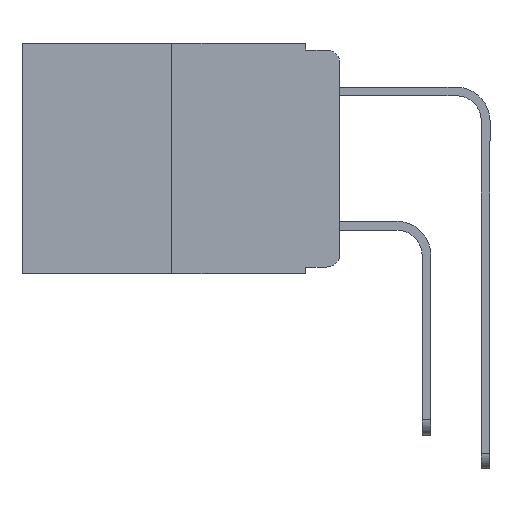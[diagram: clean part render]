
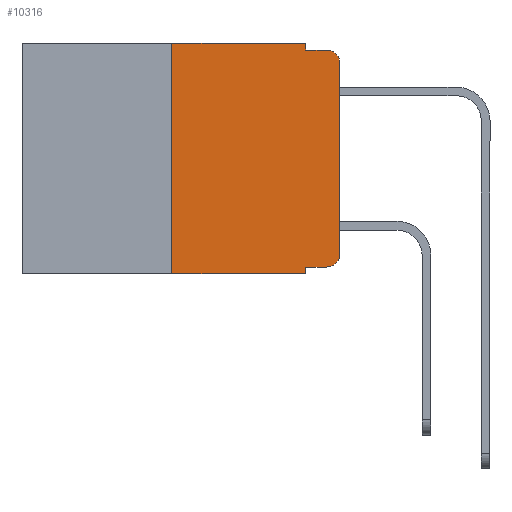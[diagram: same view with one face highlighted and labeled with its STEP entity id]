
A CAD part, left-side view. The second image highlights one B-rep face of the part: STEP entity #10316.
In plain terms, the highlighted planar face has unit normal (-1, 0, 0).
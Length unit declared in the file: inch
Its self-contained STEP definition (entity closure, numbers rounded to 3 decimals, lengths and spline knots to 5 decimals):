
#369 = LINE ( 'NONE', #493, #10922 ) ;
#422 = VERTEX_POINT ( 'NONE', #744 ) ;
#456 = CARTESIAN_POINT ( 'NONE',  ( 0., 0.051, -0.01 ) ) ;
#493 = CARTESIAN_POINT ( 'NONE',  ( 0., 0.473, 0. ) ) ;
#635 = EDGE_CURVE ( 'NONE', #11905, #3567, #12122, .T. ) ;
#669 = LINE ( 'NONE', #4053, #11160 ) ;
#709 = VERTEX_POINT ( 'NONE', #1721 ) ;
#716 = VERTEX_POINT ( 'NONE', #5108 ) ;
#744 = CARTESIAN_POINT ( 'NONE',  ( 0., 0.051, -0.343 ) ) ;
#819 = DIRECTION ( 'NONE',  ( 0., -1., 0. ) ) ;
#1115 = CARTESIAN_POINT ( 'NONE',  ( 0., 0.473, 0. ) ) ;
#1417 = DIRECTION ( 'NONE',  ( 0., 0., 1. ) ) ;
#1721 = CARTESIAN_POINT ( 'NONE',  ( 0., 0., -0.313 ) ) ;
#1828 = DIRECTION ( 'NONE',  ( 0., 0., -1. ) ) ;
#1864 = DIRECTION ( 'NONE',  ( -1., 0., 0. ) ) ;
#1918 = CARTESIAN_POINT ( 'NONE',  ( 0., 0.473, -0.343 ) ) ;
#2190 = DIRECTION ( 'NONE',  ( 0., -1., 0. ) ) ;
#2200 = PLANE ( 'NONE',  #5521 ) ;
#2297 = CIRCLE ( 'NONE', #5260, 0.02 ) ;
#2312 = VECTOR ( 'NONE', #10658, 39.37008 ) ;
#2382 = DIRECTION ( 'NONE',  ( 0., 0., -1. ) ) ;
#2563 = FACE_OUTER_BOUND ( 'NONE', #3413, .T. ) ;
#2574 = ORIENTED_EDGE ( 'NONE', *, *, #4905, .F. ) ;
#2750 = ORIENTED_EDGE ( 'NONE', *, *, #12150, .F. ) ;
#2916 = CARTESIAN_POINT ( 'NONE',  ( 0., 0.051, 0. ) ) ;
#3266 = ORIENTED_EDGE ( 'NONE', *, *, #9409, .F. ) ;
#3413 = EDGE_LOOP ( 'NONE', ( #11292, #5537, #2574, #2750, #3266, #3460, #7103, #6389, #4640, #3563 ) ) ;
#3460 = ORIENTED_EDGE ( 'NONE', *, *, #635, .F. ) ;
#3563 = ORIENTED_EDGE ( 'NONE', *, *, #5731, .T. ) ;
#3567 = VERTEX_POINT ( 'NONE', #7521 ) ;
#4053 = CARTESIAN_POINT ( 'NONE',  ( 0., 0.051, 0. ) ) ;
#4135 = LINE ( 'NONE', #1918, #9177 ) ;
#4256 = DIRECTION ( 'NONE',  ( 1., 0., 0. ) ) ;
#4304 = DIRECTION ( 'NONE',  ( 0., 0., 1. ) ) ;
#4493 = CARTESIAN_POINT ( 'NONE',  ( 0., 0.02, -0.03 ) ) ;
#4640 = ORIENTED_EDGE ( 'NONE', *, *, #7747, .T. ) ;
#4781 = DIRECTION ( 'NONE',  ( 0., -1., 0. ) ) ;
#4905 = EDGE_CURVE ( 'NONE', #8538, #7505, #7446, .T. ) ;
#5053 = CARTESIAN_POINT ( 'NONE',  ( 0., 0.02, -0.333 ) ) ;
#5089 = VECTOR ( 'NONE', #2382, 39.37008 ) ;
#5108 = CARTESIAN_POINT ( 'NONE',  ( 0., 0., -0.03 ) ) ;
#5260 = AXIS2_PLACEMENT_3D ( 'NONE', #4493, #11409, #5527 ) ;
#5336 = CARTESIAN_POINT ( 'NONE',  ( 0., 0., 0. ) ) ;
#5478 = EDGE_CURVE ( 'NONE', #12094, #422, #12902, .T. ) ;
#5521 = AXIS2_PLACEMENT_3D ( 'NONE', #1115, #4256, #9312 ) ;
#5527 = DIRECTION ( 'NONE',  ( 0., 0., -1. ) ) ;
#5537 = ORIENTED_EDGE ( 'NONE', *, *, #8377, .T. ) ;
#5731 = EDGE_CURVE ( 'NONE', #9114, #709, #10222, .T. ) ;
#6389 = ORIENTED_EDGE ( 'NONE', *, *, #5478, .F. ) ;
#6400 = CARTESIAN_POINT ( 'NONE',  ( 0., 0.02, -0.313 ) ) ;
#7103 = ORIENTED_EDGE ( 'NONE', *, *, #7580, .T. ) ;
#7446 = LINE ( 'NONE', #456, #2312 ) ;
#7505 = VERTEX_POINT ( 'NONE', #11778 ) ;
#7521 = CARTESIAN_POINT ( 'NONE',  ( 0., 0.25, 0. ) ) ;
#7556 = VERTEX_POINT ( 'NONE', #9016 ) ;
#7580 = EDGE_CURVE ( 'NONE', #11905, #422, #4135, .T. ) ;
#7747 = EDGE_CURVE ( 'NONE', #12094, #9114, #10820, .T. ) ;
#8141 = CARTESIAN_POINT ( 'NONE',  ( 0., 0.25, 0. ) ) ;
#8377 = EDGE_CURVE ( 'NONE', #716, #7505, #2297, .T. ) ;
#8538 = VERTEX_POINT ( 'NONE', #9751 ) ;
#9016 = CARTESIAN_POINT ( 'NONE',  ( 0., 0.051, 0. ) ) ;
#9114 = VERTEX_POINT ( 'NONE', #5053 ) ;
#9177 = VECTOR ( 'NONE', #819, 39.37008 ) ;
#9312 = DIRECTION ( 'NONE',  ( 0., 0., -1. ) ) ;
#9409 = EDGE_CURVE ( 'NONE', #3567, #7556, #369, .T. ) ;
#9589 = CARTESIAN_POINT ( 'NONE',  ( 0., 0.25, -0.343 ) ) ;
#9590 = VECTOR ( 'NONE', #1417, 39.37008 ) ;
#9751 = CARTESIAN_POINT ( 'NONE',  ( 0., 0.051, -0.01 ) ) ;
#9929 = VECTOR ( 'NONE', #2190, 39.37008 ) ;
#10222 = CIRCLE ( 'NONE', #11117, 0.02 ) ;
#10305 = VECTOR ( 'NONE', #4304, 39.37008 ) ;
#10316 = ADVANCED_FACE ( 'NONE', ( #2563 ), #2200, .F. ) ;
#10331 = EDGE_CURVE ( 'NONE', #709, #716, #12822, .T. ) ;
#10658 = DIRECTION ( 'NONE',  ( 0., -1., 0. ) ) ;
#10820 = LINE ( 'NONE', #13085, #9929 ) ;
#10882 = CARTESIAN_POINT ( 'NONE',  ( 0., 0.051, -0.333 ) ) ;
#10922 = VECTOR ( 'NONE', #4781, 39.37008 ) ;
#11010 = DIRECTION ( 'NONE',  ( 0., 0., -1. ) ) ;
#11117 = AXIS2_PLACEMENT_3D ( 'NONE', #6400, #1864, #1828 ) ;
#11160 = VECTOR ( 'NONE', #11010, 39.37008 ) ;
#11292 = ORIENTED_EDGE ( 'NONE', *, *, #10331, .T. ) ;
#11409 = DIRECTION ( 'NONE',  ( -1., 0., 0. ) ) ;
#11778 = CARTESIAN_POINT ( 'NONE',  ( 0., 0.02, -0.01 ) ) ;
#11905 = VERTEX_POINT ( 'NONE', #9589 ) ;
#12094 = VERTEX_POINT ( 'NONE', #10882 ) ;
#12122 = LINE ( 'NONE', #8141, #9590 ) ;
#12150 = EDGE_CURVE ( 'NONE', #7556, #8538, #669, .T. ) ;
#12822 = LINE ( 'NONE', #5336, #10305 ) ;
#12902 = LINE ( 'NONE', #2916, #5089 ) ;
#13085 = CARTESIAN_POINT ( 'NONE',  ( 0., 0.051, -0.333 ) ) ;
